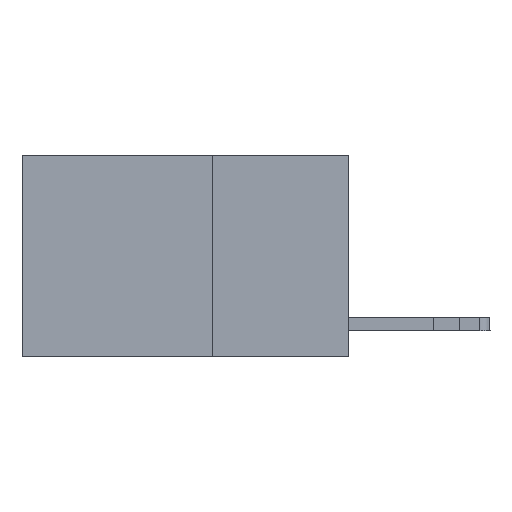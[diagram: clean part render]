
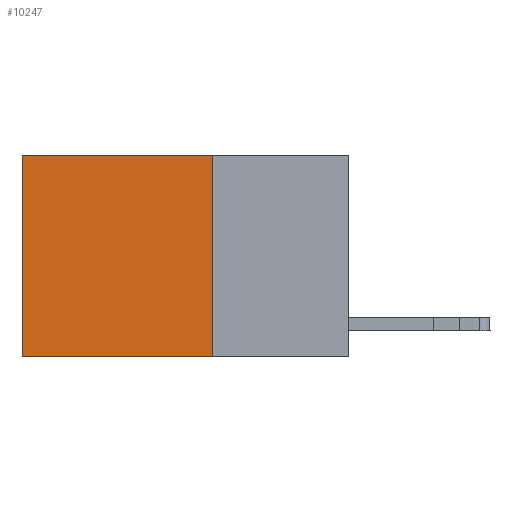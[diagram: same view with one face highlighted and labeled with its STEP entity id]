
A CAD part, left-side view. The second image highlights one B-rep face of the part: STEP entity #10247.
In plain terms, the highlighted planar face has unit normal (-1, 0, 0).
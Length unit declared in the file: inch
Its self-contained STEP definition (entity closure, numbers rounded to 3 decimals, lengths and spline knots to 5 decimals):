
#642 = VECTOR ( 'NONE', #18298, 39.37008 ) ;
#1219 = CARTESIAN_POINT ( 'NONE',  ( 0.2625, 0.6, 0. ) ) ;
#1616 = CARTESIAN_POINT ( 'NONE',  ( 0.2625, 0.25, -0.37 ) ) ;
#1696 = EDGE_CURVE ( 'NONE', #16176, #6061, #18067, .T. ) ;
#1972 = CARTESIAN_POINT ( 'NONE',  ( 0.2625, 0.25, -0.37 ) ) ;
#2312 = ORIENTED_EDGE ( 'NONE', *, *, #1696, .T. ) ;
#3145 = VERTEX_POINT ( 'NONE', #1616 ) ;
#6061 = VERTEX_POINT ( 'NONE', #9774 ) ;
#6527 = DIRECTION ( 'NONE',  ( 0., 1., 0. ) ) ;
#6642 = CARTESIAN_POINT ( 'NONE',  ( 0.2625, 0.6, 0. ) ) ;
#6751 = LINE ( 'NONE', #16922, #20392 ) ;
#6833 = CARTESIAN_POINT ( 'NONE',  ( 0.2625, 0.25, 0. ) ) ;
#8832 = DIRECTION ( 'NONE',  ( 0., 0., -1. ) ) ;
#9652 = VERTEX_POINT ( 'NONE', #6833 ) ;
#9774 = CARTESIAN_POINT ( 'NONE',  ( 0.2625, 0.6, -0.37 ) ) ;
#10247 = ADVANCED_FACE ( 'NONE', ( #19581 ), #19792, .F. ) ;
#10269 = VECTOR ( 'NONE', #8832, 39.37008 ) ;
#10436 = LINE ( 'NONE', #1972, #18605 ) ;
#11158 = EDGE_CURVE ( 'NONE', #3145, #6061, #10436, .T. ) ;
#11293 = DIRECTION ( 'NONE',  ( 1., 0., 0. ) ) ;
#11567 = ORIENTED_EDGE ( 'NONE', *, *, #11158, .F. ) ;
#12402 = LINE ( 'NONE', #16006, #10269 ) ;
#13106 = AXIS2_PLACEMENT_3D ( 'NONE', #17823, #11293, #18026 ) ;
#14232 = DIRECTION ( 'NONE',  ( 0., 1., 0. ) ) ;
#16006 = CARTESIAN_POINT ( 'NONE',  ( 0.2625, 0.25, 0. ) ) ;
#16176 = VERTEX_POINT ( 'NONE', #6642 ) ;
#16626 = EDGE_LOOP ( 'NONE', ( #2312, #11567, #19788, #19208 ) ) ;
#16922 = CARTESIAN_POINT ( 'NONE',  ( 0.2625, 0.25, 0. ) ) ;
#16929 = EDGE_CURVE ( 'NONE', #9652, #3145, #12402, .T. ) ;
#17823 = CARTESIAN_POINT ( 'NONE',  ( 0.2625, 0.25, 0. ) ) ;
#18026 = DIRECTION ( 'NONE',  ( 0., 0., -1. ) ) ;
#18067 = LINE ( 'NONE', #1219, #642 ) ;
#18298 = DIRECTION ( 'NONE',  ( 0., 0., -1. ) ) ;
#18605 = VECTOR ( 'NONE', #14232, 39.37008 ) ;
#19208 = ORIENTED_EDGE ( 'NONE', *, *, #21229, .T. ) ;
#19581 = FACE_OUTER_BOUND ( 'NONE', #16626, .T. ) ;
#19788 = ORIENTED_EDGE ( 'NONE', *, *, #16929, .F. ) ;
#19792 = PLANE ( 'NONE',  #13106 ) ;
#20392 = VECTOR ( 'NONE', #6527, 39.37008 ) ;
#21229 = EDGE_CURVE ( 'NONE', #9652, #16176, #6751, .T. ) ;
